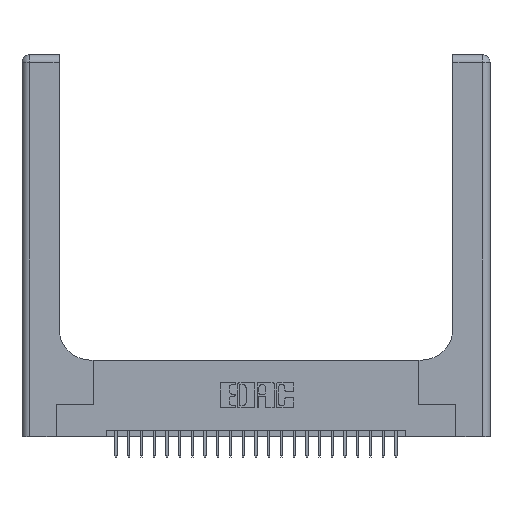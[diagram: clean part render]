
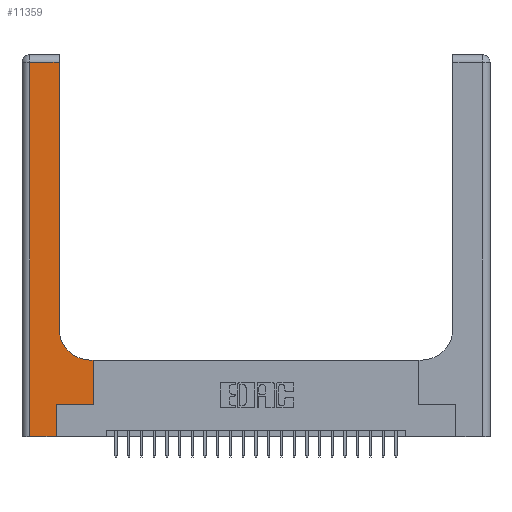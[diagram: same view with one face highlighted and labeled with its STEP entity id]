
A CAD part, top view. The second image highlights one B-rep face of the part: STEP entity #11359.
In plain terms, the highlighted planar face has unit normal (0, 0, 1).
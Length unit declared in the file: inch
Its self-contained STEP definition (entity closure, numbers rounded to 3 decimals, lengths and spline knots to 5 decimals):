
#318 = EDGE_CURVE ( 'NONE', #7358, #7351, #7403, .T. ) ;
#714 = CARTESIAN_POINT ( 'NONE',  ( 0.2915, 2.94, 0.37 ) ) ;
#1138 = DIRECTION ( 'NONE',  ( 1., 0., 0. ) ) ;
#1429 = AXIS2_PLACEMENT_3D ( 'NONE', #18458, #6419, #20432 ) ;
#1615 = DIRECTION ( 'NONE',  ( 1., 0., 0. ) ) ;
#1741 = DIRECTION ( 'NONE',  ( 0., 1., 0. ) ) ;
#1767 = LINE ( 'NONE', #25662, #11229 ) ;
#2097 = VERTEX_POINT ( 'NONE', #22684 ) ;
#2698 = DIRECTION ( 'NONE',  ( -1., 0., 0. ) ) ;
#3724 = LINE ( 'NONE', #14145, #23125 ) ;
#3743 = ORIENTED_EDGE ( 'NONE', *, *, #22607, .T. ) ;
#4014 = DIRECTION ( 'NONE',  ( 0., 1., 0. ) ) ;
#4869 = VERTEX_POINT ( 'NONE', #6749 ) ;
#4960 = LINE ( 'NONE', #16826, #15665 ) ;
#5373 = CARTESIAN_POINT ( 'NONE',  ( 0.269, 0.25, 0.37 ) ) ;
#5788 = ORIENTED_EDGE ( 'NONE', *, *, #18057, .T. ) ;
#6163 = EDGE_CURVE ( 'NONE', #6362, #2097, #4960, .T. ) ;
#6362 = VERTEX_POINT ( 'NONE', #9231 ) ;
#6419 = DIRECTION ( 'NONE',  ( 0., 0., -1. ) ) ;
#6622 = EDGE_CURVE ( 'NONE', #11393, #7120, #11527, .T. ) ;
#6749 = CARTESIAN_POINT ( 'NONE',  ( 0.5585, 0.25, 0.37 ) ) ;
#6978 = EDGE_CURVE ( 'NONE', #7351, #11393, #22750, .T. ) ;
#7120 = VERTEX_POINT ( 'NONE', #5373 ) ;
#7351 = VERTEX_POINT ( 'NONE', #20111 ) ;
#7358 = VERTEX_POINT ( 'NONE', #22163 ) ;
#7403 = LINE ( 'NONE', #15787, #17484 ) ;
#7971 = EDGE_LOOP ( 'NONE', ( #13999, #3743, #21583, #14521, #9583, #16455, #23012, #20367, #5788 ) ) ;
#9231 = CARTESIAN_POINT ( 'NONE',  ( 0.5585, 0.6, 0.37 ) ) ;
#9583 = ORIENTED_EDGE ( 'NONE', *, *, #6622, .T. ) ;
#10029 = CARTESIAN_POINT ( 'NONE',  ( 0.269, 0., 0.37 ) ) ;
#10626 = LINE ( 'NONE', #17184, #25214 ) ;
#11229 = VECTOR ( 'NONE', #1741, 39.37008 ) ;
#11359 = ADVANCED_FACE ( 'NONE', ( #19188 ), #14425, .F. ) ;
#11393 = VERTEX_POINT ( 'NONE', #14602 ) ;
#11527 = LINE ( 'NONE', #10029, #15644 ) ;
#12166 = VECTOR ( 'NONE', #22942, 39.37008 ) ;
#12399 = VECTOR ( 'NONE', #23148, 39.37008 ) ;
#12729 = CARTESIAN_POINT ( 'NONE',  ( 0.2915, 0.85, 0.37 ) ) ;
#13572 = EDGE_CURVE ( 'NONE', #17741, #23078, #1767, .T. ) ;
#13696 = DIRECTION ( 'NONE',  ( 0., 0., -1. ) ) ;
#13999 = ORIENTED_EDGE ( 'NONE', *, *, #13572, .T. ) ;
#14145 = CARTESIAN_POINT ( 'NONE',  ( 0.5585, 0.25, 0.37 ) ) ;
#14425 = PLANE ( 'NONE',  #1429 ) ;
#14521 = ORIENTED_EDGE ( 'NONE', *, *, #6978, .T. ) ;
#14602 = CARTESIAN_POINT ( 'NONE',  ( 0.269, 0., 0.37 ) ) ;
#15525 = DIRECTION ( 'NONE',  ( 0., -1., 0. ) ) ;
#15644 = VECTOR ( 'NONE', #4014, 39.37008 ) ;
#15665 = VECTOR ( 'NONE', #2698, 39.37008 ) ;
#15787 = CARTESIAN_POINT ( 'NONE',  ( 0.06, 3., 0.37 ) ) ;
#16455 = ORIENTED_EDGE ( 'NONE', *, *, #20873, .T. ) ;
#16688 = CIRCLE ( 'NONE', #24625, 0.25 ) ;
#16826 = CARTESIAN_POINT ( 'NONE',  ( 0.2915, 0.6, 0.37 ) ) ;
#17184 = CARTESIAN_POINT ( 'NONE',  ( 0.269, 0.25, 0.37 ) ) ;
#17484 = VECTOR ( 'NONE', #15525, 39.37008 ) ;
#17741 = VERTEX_POINT ( 'NONE', #12729 ) ;
#18057 = EDGE_CURVE ( 'NONE', #2097, #17741, #16688, .T. ) ;
#18187 = DIRECTION ( 'NONE',  ( 0., 1., 0. ) ) ;
#18458 = CARTESIAN_POINT ( 'NONE',  ( 0., 3., 0.37 ) ) ;
#18918 = CARTESIAN_POINT ( 'NONE',  ( 0., 0., 0.37 ) ) ;
#19188 = FACE_OUTER_BOUND ( 'NONE', #7971, .T. ) ;
#20111 = CARTESIAN_POINT ( 'NONE',  ( 0.06, 0., 0.37 ) ) ;
#20367 = ORIENTED_EDGE ( 'NONE', *, *, #6163, .T. ) ;
#20432 = DIRECTION ( 'NONE',  ( -1., 0., 0. ) ) ;
#20873 = EDGE_CURVE ( 'NONE', #7120, #4869, #10626, .T. ) ;
#21583 = ORIENTED_EDGE ( 'NONE', *, *, #318, .T. ) ;
#22163 = CARTESIAN_POINT ( 'NONE',  ( 0.06, 2.94, 0.37 ) ) ;
#22607 = EDGE_CURVE ( 'NONE', #23078, #7358, #22976, .T. ) ;
#22684 = CARTESIAN_POINT ( 'NONE',  ( 0.5415, 0.6, 0.37 ) ) ;
#22750 = LINE ( 'NONE', #18918, #12166 ) ;
#22942 = DIRECTION ( 'NONE',  ( 1., 0., 0. ) ) ;
#22976 = LINE ( 'NONE', #25119, #12399 ) ;
#23012 = ORIENTED_EDGE ( 'NONE', *, *, #25566, .T. ) ;
#23078 = VERTEX_POINT ( 'NONE', #714 ) ;
#23125 = VECTOR ( 'NONE', #18187, 39.37008 ) ;
#23148 = DIRECTION ( 'NONE',  ( -1., 0., 0. ) ) ;
#24625 = AXIS2_PLACEMENT_3D ( 'NONE', #25541, #13696, #1615 ) ;
#25119 = CARTESIAN_POINT ( 'NONE',  ( 0., 2.94, 0.37 ) ) ;
#25214 = VECTOR ( 'NONE', #1138, 39.37008 ) ;
#25541 = CARTESIAN_POINT ( 'NONE',  ( 0.5415, 0.85, 0.37 ) ) ;
#25566 = EDGE_CURVE ( 'NONE', #4869, #6362, #3724, .T. ) ;
#25662 = CARTESIAN_POINT ( 'NONE',  ( 0.2915, 3., 0.37 ) ) ;
